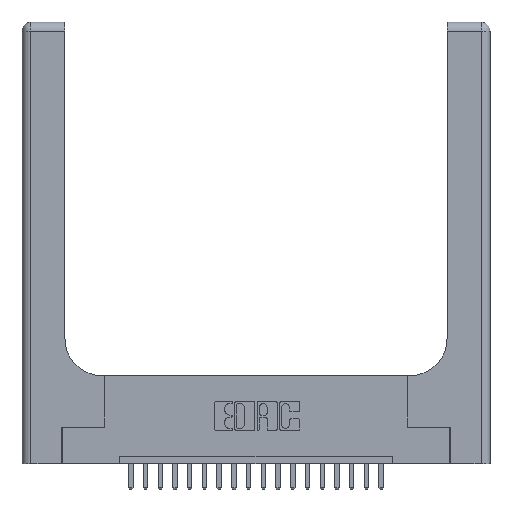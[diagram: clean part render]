
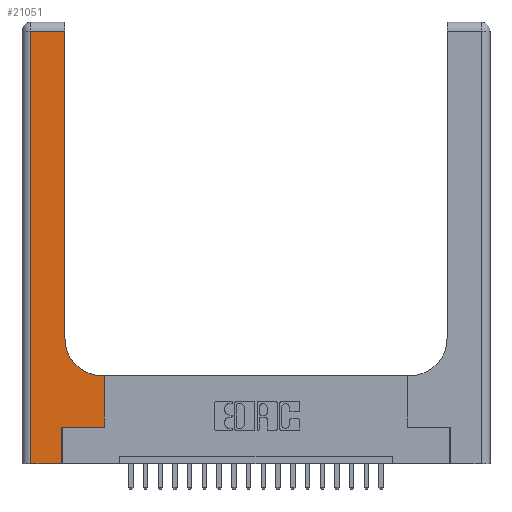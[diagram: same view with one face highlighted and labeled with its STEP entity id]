
A CAD part, top view. The second image highlights one B-rep face of the part: STEP entity #21051.
In plain terms, the highlighted planar face has unit normal (0, 0, 1).
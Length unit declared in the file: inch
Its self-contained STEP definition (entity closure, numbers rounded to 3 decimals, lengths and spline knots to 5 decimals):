
#563 = ORIENTED_EDGE ( 'NONE', *, *, #15945, .T. ) ;
#716 = LINE ( 'NONE', #12847, #2596 ) ;
#1530 = LINE ( 'NONE', #21373, #7912 ) ;
#1772 = AXIS2_PLACEMENT_3D ( 'NONE', #7118, #5636, #19125 ) ;
#1873 = CARTESIAN_POINT ( 'NONE',  ( 0.5415, 0.6, 0.37 ) ) ;
#2223 = ORIENTED_EDGE ( 'NONE', *, *, #10617, .T. ) ;
#2267 = CIRCLE ( 'NONE', #1772, 0.25 ) ;
#2560 = CARTESIAN_POINT ( 'NONE',  ( 0.2915, 3., 0.37 ) ) ;
#2567 = ORIENTED_EDGE ( 'NONE', *, *, #20511, .T. ) ;
#2596 = VECTOR ( 'NONE', #6007, 39.37008 ) ;
#2856 = EDGE_LOOP ( 'NONE', ( #2567, #15078, #7168, #8740, #12533, #4567, #2223, #18970, #563 ) ) ;
#2979 = EDGE_CURVE ( 'NONE', #4225, #21396, #10670, .T. ) ;
#3172 = CARTESIAN_POINT ( 'NONE',  ( 0.269, 0., 0.37 ) ) ;
#3815 = LINE ( 'NONE', #2560, #9143 ) ;
#4056 = LINE ( 'NONE', #10193, #20333 ) ;
#4225 = VERTEX_POINT ( 'NONE', #10174 ) ;
#4292 = EDGE_CURVE ( 'NONE', #19760, #4225, #20227, .T. ) ;
#4567 = ORIENTED_EDGE ( 'NONE', *, *, #17599, .T. ) ;
#4993 = VERTEX_POINT ( 'NONE', #20561 ) ;
#5014 = VERTEX_POINT ( 'NONE', #1873 ) ;
#5636 = DIRECTION ( 'NONE',  ( 0., 0., -1. ) ) ;
#6007 = DIRECTION ( 'NONE',  ( -1., 0., 0. ) ) ;
#6098 = VERTEX_POINT ( 'NONE', #13512 ) ;
#6254 = AXIS2_PLACEMENT_3D ( 'NONE', #16135, #7646, #17930 ) ;
#6476 = CARTESIAN_POINT ( 'NONE',  ( 0., 0., 0.37 ) ) ;
#6622 = VECTOR ( 'NONE', #11938, 39.37008 ) ;
#7118 = CARTESIAN_POINT ( 'NONE',  ( 0.5415, 0.85, 0.37 ) ) ;
#7168 = ORIENTED_EDGE ( 'NONE', *, *, #4292, .T. ) ;
#7646 = DIRECTION ( 'NONE',  ( 0., 0., -1. ) ) ;
#7912 = VECTOR ( 'NONE', #9769, 39.37008 ) ;
#8204 = CARTESIAN_POINT ( 'NONE',  ( 0.2915, 2.94, 0.37 ) ) ;
#8235 = DIRECTION ( 'NONE',  ( 0., 1., 0. ) ) ;
#8471 = VECTOR ( 'NONE', #14282, 39.37008 ) ;
#8740 = ORIENTED_EDGE ( 'NONE', *, *, #2979, .T. ) ;
#8859 = FACE_OUTER_BOUND ( 'NONE', #2856, .T. ) ;
#9094 = CARTESIAN_POINT ( 'NONE',  ( 0., 2.94, 0.37 ) ) ;
#9143 = VECTOR ( 'NONE', #9479, 39.37008 ) ;
#9479 = DIRECTION ( 'NONE',  ( 0., 1., 0. ) ) ;
#9769 = DIRECTION ( 'NONE',  ( 1., 0., 0. ) ) ;
#9901 = VECTOR ( 'NONE', #14895, 39.37008 ) ;
#10089 = VECTOR ( 'NONE', #11341, 39.37008 ) ;
#10174 = CARTESIAN_POINT ( 'NONE',  ( 0.06, 0., 0.37 ) ) ;
#10193 = CARTESIAN_POINT ( 'NONE',  ( 0.5585, 0.25, 0.37 ) ) ;
#10337 = LINE ( 'NONE', #9094, #8471 ) ;
#10617 = EDGE_CURVE ( 'NONE', #4993, #6098, #4056, .T. ) ;
#10670 = LINE ( 'NONE', #6476, #9901 ) ;
#10774 = CARTESIAN_POINT ( 'NONE',  ( 0.06, 2.94, 0.37 ) ) ;
#11341 = DIRECTION ( 'NONE',  ( 0., 1., 0. ) ) ;
#11938 = DIRECTION ( 'NONE',  ( 0., -1., 0. ) ) ;
#12038 = VERTEX_POINT ( 'NONE', #19887 ) ;
#12533 = ORIENTED_EDGE ( 'NONE', *, *, #16978, .T. ) ;
#12847 = CARTESIAN_POINT ( 'NONE',  ( 0.2915, 0.6, 0.37 ) ) ;
#13389 = EDGE_CURVE ( 'NONE', #16898, #19760, #10337, .T. ) ;
#13512 = CARTESIAN_POINT ( 'NONE',  ( 0.5585, 0.6, 0.37 ) ) ;
#13817 = CARTESIAN_POINT ( 'NONE',  ( 0.269, 0., 0.37 ) ) ;
#14282 = DIRECTION ( 'NONE',  ( -1., 0., 0. ) ) ;
#14895 = DIRECTION ( 'NONE',  ( 1., 0., 0. ) ) ;
#15078 = ORIENTED_EDGE ( 'NONE', *, *, #13389, .T. ) ;
#15296 = CARTESIAN_POINT ( 'NONE',  ( 0.06, 3., 0.37 ) ) ;
#15945 = EDGE_CURVE ( 'NONE', #5014, #12038, #2267, .T. ) ;
#16135 = CARTESIAN_POINT ( 'NONE',  ( 0., 3., 0.37 ) ) ;
#16898 = VERTEX_POINT ( 'NONE', #8204 ) ;
#16978 = EDGE_CURVE ( 'NONE', #21396, #17426, #21265, .T. ) ;
#17239 = EDGE_CURVE ( 'NONE', #6098, #5014, #716, .T. ) ;
#17426 = VERTEX_POINT ( 'NONE', #19156 ) ;
#17599 = EDGE_CURVE ( 'NONE', #17426, #4993, #1530, .T. ) ;
#17930 = DIRECTION ( 'NONE',  ( -1., 0., 0. ) ) ;
#18970 = ORIENTED_EDGE ( 'NONE', *, *, #17239, .T. ) ;
#19125 = DIRECTION ( 'NONE',  ( 1., 0., 0. ) ) ;
#19156 = CARTESIAN_POINT ( 'NONE',  ( 0.269, 0.25, 0.37 ) ) ;
#19760 = VERTEX_POINT ( 'NONE', #10774 ) ;
#19808 = PLANE ( 'NONE',  #6254 ) ;
#19887 = CARTESIAN_POINT ( 'NONE',  ( 0.2915, 0.85, 0.37 ) ) ;
#20227 = LINE ( 'NONE', #15296, #6622 ) ;
#20333 = VECTOR ( 'NONE', #8235, 39.37008 ) ;
#20511 = EDGE_CURVE ( 'NONE', #12038, #16898, #3815, .T. ) ;
#20561 = CARTESIAN_POINT ( 'NONE',  ( 0.5585, 0.25, 0.37 ) ) ;
#21051 = ADVANCED_FACE ( 'NONE', ( #8859 ), #19808, .F. ) ;
#21265 = LINE ( 'NONE', #3172, #10089 ) ;
#21373 = CARTESIAN_POINT ( 'NONE',  ( 0.269, 0.25, 0.37 ) ) ;
#21396 = VERTEX_POINT ( 'NONE', #13817 ) ;
